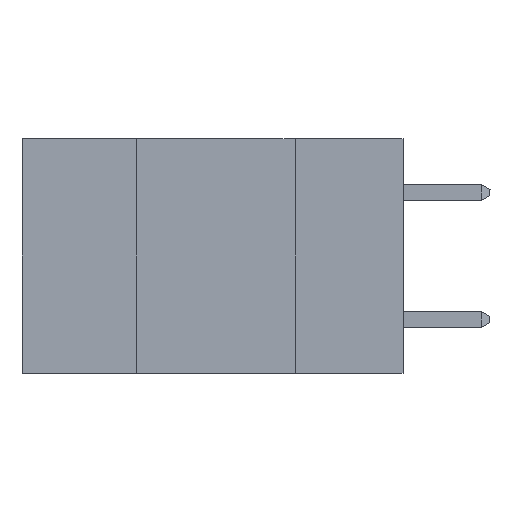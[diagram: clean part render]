
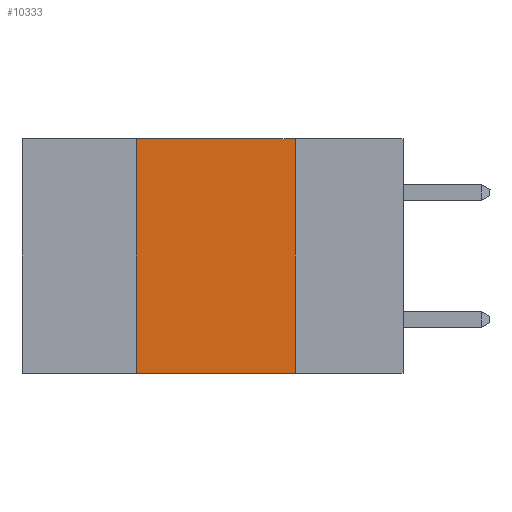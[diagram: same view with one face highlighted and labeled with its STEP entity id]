
A CAD part, left-side view. The second image highlights one B-rep face of the part: STEP entity #10333.
In plain terms, the highlighted planar face has unit normal (-1, 0, 0).
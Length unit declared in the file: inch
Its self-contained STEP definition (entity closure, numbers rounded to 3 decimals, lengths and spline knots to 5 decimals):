
#65 = ORIENTED_EDGE ( 'NONE', *, *, #16188, .T. ) ;
#125 = FACE_OUTER_BOUND ( 'NONE', #382, .T. ) ;
#382 = EDGE_LOOP ( 'NONE', ( #13357, #18260, #6156, #65 ) ) ;
#954 = CARTESIAN_POINT ( 'NONE',  ( 0., 0.42, 0. ) ) ;
#2098 = CARTESIAN_POINT ( 'NONE',  ( 0., 0.42, -0.37 ) ) ;
#3109 = DIRECTION ( 'NONE',  ( 0., 0., -1. ) ) ;
#4195 = LINE ( 'NONE', #22537, #18143 ) ;
#4216 = EDGE_CURVE ( 'NONE', #21548, #21910, #7909, .T. ) ;
#5136 = AXIS2_PLACEMENT_3D ( 'NONE', #17904, #8838, #17591 ) ;
#6156 = ORIENTED_EDGE ( 'NONE', *, *, #15664, .F. ) ;
#6753 = VECTOR ( 'NONE', #7847, 39.37008 ) ;
#6982 = EDGE_CURVE ( 'NONE', #14193, #21548, #4195, .T. ) ;
#7108 = VERTEX_POINT ( 'NONE', #2098 ) ;
#7847 = DIRECTION ( 'NONE',  ( 0., -1., 0. ) ) ;
#7849 = LINE ( 'NONE', #17096, #17960 ) ;
#7909 = LINE ( 'NONE', #17898, #9000 ) ;
#8838 = DIRECTION ( 'NONE',  ( 1., 0., 0. ) ) ;
#9000 = VECTOR ( 'NONE', #3109, 39.37008 ) ;
#10253 = DIRECTION ( 'NONE',  ( 0., 0., 1. ) ) ;
#10333 = ADVANCED_FACE ( 'NONE', ( #125 ), #12644, .F. ) ;
#12644 = PLANE ( 'NONE',  #5136 ) ;
#13122 = CARTESIAN_POINT ( 'NONE',  ( 0., 0.6, -0.37 ) ) ;
#13357 = ORIENTED_EDGE ( 'NONE', *, *, #4216, .F. ) ;
#14193 = VERTEX_POINT ( 'NONE', #954 ) ;
#14294 = CARTESIAN_POINT ( 'NONE',  ( 0., 0.17, 0. ) ) ;
#14904 = CARTESIAN_POINT ( 'NONE',  ( 0., 0.17, -0.37 ) ) ;
#15664 = EDGE_CURVE ( 'NONE', #7108, #14193, #7849, .T. ) ;
#16188 = EDGE_CURVE ( 'NONE', #7108, #21910, #21997, .T. ) ;
#17096 = CARTESIAN_POINT ( 'NONE',  ( 0., 0.42, 0. ) ) ;
#17366 = DIRECTION ( 'NONE',  ( 0., -1., 0. ) ) ;
#17591 = DIRECTION ( 'NONE',  ( 0., 0., -1. ) ) ;
#17898 = CARTESIAN_POINT ( 'NONE',  ( 0., 0.17, 0. ) ) ;
#17904 = CARTESIAN_POINT ( 'NONE',  ( 0., 0.6, 0. ) ) ;
#17960 = VECTOR ( 'NONE', #10253, 39.37008 ) ;
#18143 = VECTOR ( 'NONE', #17366, 39.37008 ) ;
#18260 = ORIENTED_EDGE ( 'NONE', *, *, #6982, .F. ) ;
#21548 = VERTEX_POINT ( 'NONE', #14294 ) ;
#21910 = VERTEX_POINT ( 'NONE', #14904 ) ;
#21997 = LINE ( 'NONE', #13122, #6753 ) ;
#22537 = CARTESIAN_POINT ( 'NONE',  ( 0., 0.6, 0. ) ) ;
